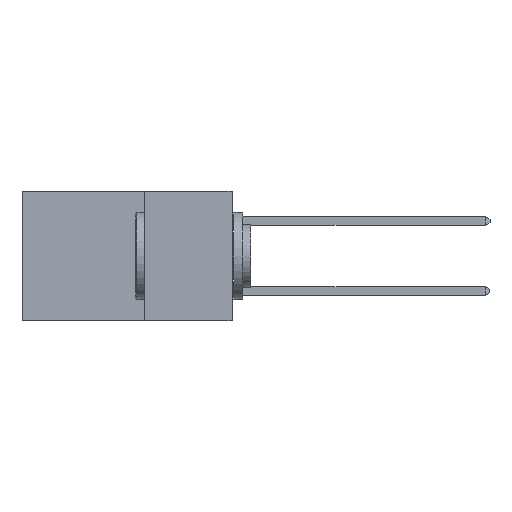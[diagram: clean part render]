
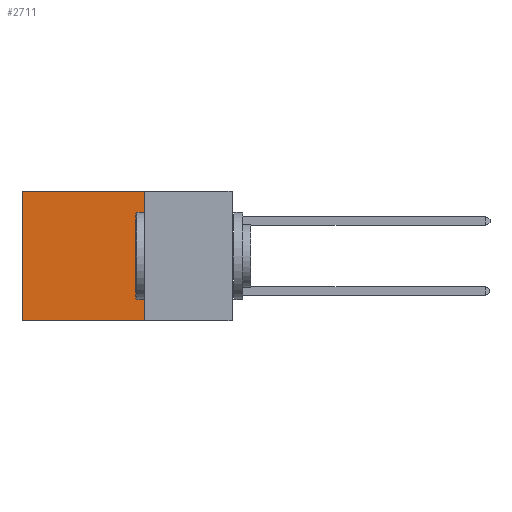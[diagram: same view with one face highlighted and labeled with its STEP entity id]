
A CAD part, left-side view. The second image highlights one B-rep face of the part: STEP entity #2711.
In plain terms, the highlighted planar face has unit normal (-1, 0, 0).
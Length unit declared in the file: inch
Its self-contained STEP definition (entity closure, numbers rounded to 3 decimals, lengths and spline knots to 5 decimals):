
#1001 = LINE ( 'NONE', #15201, #5494 ) ;
#1096 = CARTESIAN_POINT ( 'NONE',  ( 0.2875, 0.6, 0. ) ) ;
#1180 = LINE ( 'NONE', #2032, #8255 ) ;
#1615 = CARTESIAN_POINT ( 'NONE',  ( 0.2875, 0.6, -0.37 ) ) ;
#1766 = VERTEX_POINT ( 'NONE', #9154 ) ;
#2032 = CARTESIAN_POINT ( 'NONE',  ( 0.2875, 0.6, 0. ) ) ;
#2711 = ADVANCED_FACE ( 'NONE', ( #13604 ), #14718, .F. ) ;
#2779 = VERTEX_POINT ( 'NONE', #12606 ) ;
#2943 = VECTOR ( 'NONE', #14073, 39.37008 ) ;
#3445 = ORIENTED_EDGE ( 'NONE', *, *, #7145, .F. ) ;
#4069 = EDGE_CURVE ( 'NONE', #2779, #15115, #8182, .T. ) ;
#4126 = EDGE_LOOP ( 'NONE', ( #15542, #3445, #6643, #9623 ) ) ;
#4745 = VECTOR ( 'NONE', #7479, 39.37008 ) ;
#5494 = VECTOR ( 'NONE', #8442, 39.37008 ) ;
#6114 = DIRECTION ( 'NONE',  ( 0., 0., -1. ) ) ;
#6643 = ORIENTED_EDGE ( 'NONE', *, *, #9907, .F. ) ;
#7145 = EDGE_CURVE ( 'NONE', #1766, #12855, #15003, .T. ) ;
#7376 = AXIS2_PLACEMENT_3D ( 'NONE', #14290, #14261, #14234 ) ;
#7479 = DIRECTION ( 'NONE',  ( 0., 1., 0. ) ) ;
#7557 = CARTESIAN_POINT ( 'NONE',  ( 0.2875, 0.25, 0. ) ) ;
#8182 = LINE ( 'NONE', #7557, #4745 ) ;
#8255 = VECTOR ( 'NONE', #6114, 39.37008 ) ;
#8442 = DIRECTION ( 'NONE',  ( 0., 0., -1. ) ) ;
#9154 = CARTESIAN_POINT ( 'NONE',  ( 0.2875, 0.25, -0.37 ) ) ;
#9551 = CARTESIAN_POINT ( 'NONE',  ( 0.2875, 0.25, -0.37 ) ) ;
#9623 = ORIENTED_EDGE ( 'NONE', *, *, #4069, .T. ) ;
#9907 = EDGE_CURVE ( 'NONE', #2779, #1766, #1001, .T. ) ;
#10560 = EDGE_CURVE ( 'NONE', #15115, #12855, #1180, .T. ) ;
#12606 = CARTESIAN_POINT ( 'NONE',  ( 0.2875, 0.25, 0. ) ) ;
#12855 = VERTEX_POINT ( 'NONE', #1615 ) ;
#13604 = FACE_OUTER_BOUND ( 'NONE', #4126, .T. ) ;
#14073 = DIRECTION ( 'NONE',  ( 0., 1., 0. ) ) ;
#14234 = DIRECTION ( 'NONE',  ( 0., 0., -1. ) ) ;
#14261 = DIRECTION ( 'NONE',  ( 1., 0., 0. ) ) ;
#14290 = CARTESIAN_POINT ( 'NONE',  ( 0.2875, 0.25, 0. ) ) ;
#14718 = PLANE ( 'NONE',  #7376 ) ;
#15003 = LINE ( 'NONE', #9551, #2943 ) ;
#15115 = VERTEX_POINT ( 'NONE', #1096 ) ;
#15201 = CARTESIAN_POINT ( 'NONE',  ( 0.2875, 0.25, 0. ) ) ;
#15542 = ORIENTED_EDGE ( 'NONE', *, *, #10560, .T. ) ;
